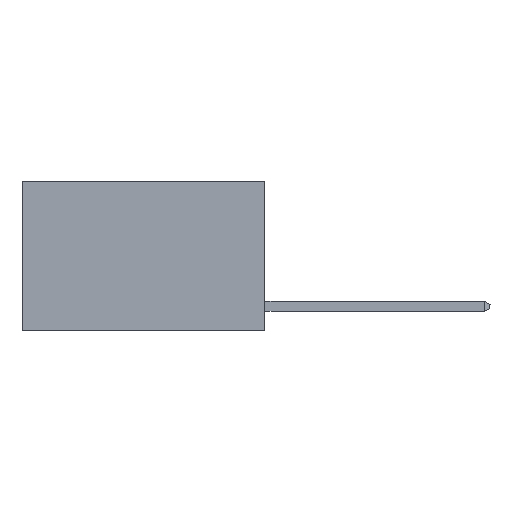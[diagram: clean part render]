
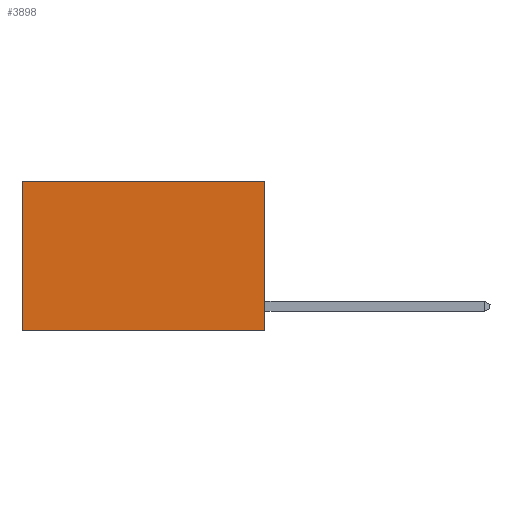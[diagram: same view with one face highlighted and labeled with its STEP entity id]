
A CAD part, left-side view. The second image highlights one B-rep face of the part: STEP entity #3898.
In plain terms, the highlighted planar face has unit normal (-1, 0, 0).
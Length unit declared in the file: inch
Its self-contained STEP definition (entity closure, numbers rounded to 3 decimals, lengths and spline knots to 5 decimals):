
#1433 = DIRECTION ( 'NONE',  ( 0., 0., -1. ) ) ;
#2173 = CARTESIAN_POINT ( 'NONE',  ( 0.2625, 0., -0.37 ) ) ;
#2636 = CARTESIAN_POINT ( 'NONE',  ( 0.2625, 0., 0. ) ) ;
#2673 = LINE ( 'NONE', #24370, #12350 ) ;
#3445 = EDGE_CURVE ( 'NONE', #9919, #21421, #13117, .T. ) ;
#3898 = ADVANCED_FACE ( 'NONE', ( #23158 ), #20053, .F. ) ;
#4399 = EDGE_CURVE ( 'NONE', #5941, #21421, #21371, .T. ) ;
#4792 = CARTESIAN_POINT ( 'NONE',  ( 0.2625, 0., 0. ) ) ;
#5941 = VERTEX_POINT ( 'NONE', #2173 ) ;
#6243 = CARTESIAN_POINT ( 'NONE',  ( 0.2625, 0., -0.37 ) ) ;
#7689 = ORIENTED_EDGE ( 'NONE', *, *, #4399, .F. ) ;
#8038 = CARTESIAN_POINT ( 'NONE',  ( 0.2625, 0., 0. ) ) ;
#8060 = ORIENTED_EDGE ( 'NONE', *, *, #17719, .F. ) ;
#8212 = DIRECTION ( 'NONE',  ( 0., 1., 0. ) ) ;
#9919 = VERTEX_POINT ( 'NONE', #12343 ) ;
#10001 = DIRECTION ( 'NONE',  ( 0., 1., 0. ) ) ;
#10226 = CARTESIAN_POINT ( 'NONE',  ( 0.2625, 0.6, -0.37 ) ) ;
#10610 = DIRECTION ( 'NONE',  ( 0., 0., -1. ) ) ;
#10696 = VECTOR ( 'NONE', #8212, 39.37008 ) ;
#12343 = CARTESIAN_POINT ( 'NONE',  ( 0.2625, 0.6, 0. ) ) ;
#12350 = VECTOR ( 'NONE', #1433, 39.37008 ) ;
#13117 = LINE ( 'NONE', #16715, #17568 ) ;
#13607 = EDGE_CURVE ( 'NONE', #23332, #9919, #24072, .T. ) ;
#16715 = CARTESIAN_POINT ( 'NONE',  ( 0.2625, 0.6, 0. ) ) ;
#17568 = VECTOR ( 'NONE', #24133, 39.37008 ) ;
#17719 = EDGE_CURVE ( 'NONE', #23332, #5941, #2673, .T. ) ;
#19011 = VECTOR ( 'NONE', #10001, 39.37008 ) ;
#19030 = ORIENTED_EDGE ( 'NONE', *, *, #13607, .T. ) ;
#20050 = EDGE_LOOP ( 'NONE', ( #22172, #7689, #8060, #19030 ) ) ;
#20053 = PLANE ( 'NONE',  #24405 ) ;
#21371 = LINE ( 'NONE', #6243, #10696 ) ;
#21421 = VERTEX_POINT ( 'NONE', #10226 ) ;
#21952 = DIRECTION ( 'NONE',  ( 1., 0., 0. ) ) ;
#22172 = ORIENTED_EDGE ( 'NONE', *, *, #3445, .T. ) ;
#23158 = FACE_OUTER_BOUND ( 'NONE', #20050, .T. ) ;
#23332 = VERTEX_POINT ( 'NONE', #4792 ) ;
#24072 = LINE ( 'NONE', #8038, #19011 ) ;
#24133 = DIRECTION ( 'NONE',  ( 0., 0., -1. ) ) ;
#24370 = CARTESIAN_POINT ( 'NONE',  ( 0.2625, 0., 0. ) ) ;
#24405 = AXIS2_PLACEMENT_3D ( 'NONE', #2636, #21952, #10610 ) ;
